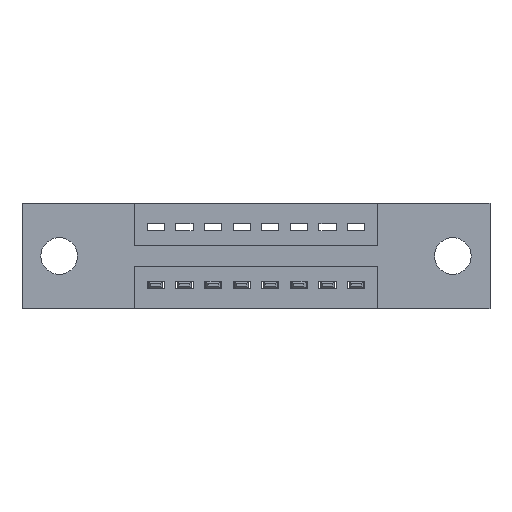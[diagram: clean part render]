
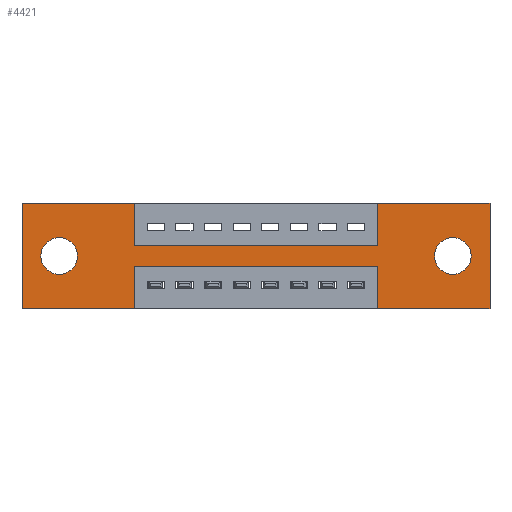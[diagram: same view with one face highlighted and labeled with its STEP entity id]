
A CAD part, front view. The second image highlights one B-rep face of the part: STEP entity #4421.
In plain terms, the highlighted planar face has unit normal (0, -1, 0).
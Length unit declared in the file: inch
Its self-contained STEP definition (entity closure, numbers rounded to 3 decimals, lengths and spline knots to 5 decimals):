
#73 = EDGE_CURVE ( 'NONE', #10025, #8509, #4733, .T. ) ;
#220 = LINE ( 'NONE', #9165, #4838 ) ;
#269 = VECTOR ( 'NONE', #8392, 39.37008 ) ;
#322 = VERTEX_POINT ( 'NONE', #3657 ) ;
#391 = CARTESIAN_POINT ( 'NONE',  ( 1.505, 0., -0.121 ) ) ;
#404 = DIRECTION ( 'NONE',  ( 0., 0., -1. ) ) ;
#452 = CARTESIAN_POINT ( 'NONE',  ( 0.3925, 0., -0.22 ) ) ;
#542 = CARTESIAN_POINT ( 'NONE',  ( 1.505, 0., -0.185 ) ) ;
#641 = DIRECTION ( 'NONE',  ( 0., 1., 0. ) ) ;
#740 = DIRECTION ( 'NONE',  ( 0., 1., 0. ) ) ;
#935 = CARTESIAN_POINT ( 'NONE',  ( 0.13, 0., -0.185 ) ) ;
#947 = EDGE_LOOP ( 'NONE', ( #5381, #6802 ) ) ;
#1046 = EDGE_CURVE ( 'NONE', #4358, #2756, #7135, .T. ) ;
#1125 = DIRECTION ( 'NONE',  ( 1., 0., 0. ) ) ;
#1167 = ORIENTED_EDGE ( 'NONE', *, *, #4762, .F. ) ;
#1325 = EDGE_LOOP ( 'NONE', ( #3595, #9137, #6911, #9579, #1167, #4138, #9545, #3908, #5271, #3804, #4996, #5662 ) ) ;
#1369 = LINE ( 'NONE', #5458, #9127 ) ;
#1416 = CARTESIAN_POINT ( 'NONE',  ( 1.635, 0., 0. ) ) ;
#1525 = CARTESIAN_POINT ( 'NONE',  ( 0.3925, 0., 0. ) ) ;
#1591 = VERTEX_POINT ( 'NONE', #1525 ) ;
#1653 = VERTEX_POINT ( 'NONE', #391 ) ;
#1808 = AXIS2_PLACEMENT_3D ( 'NONE', #6473, #740, #6333 ) ;
#1880 = VERTEX_POINT ( 'NONE', #6516 ) ;
#2045 = LINE ( 'NONE', #452, #269 ) ;
#2069 = FACE_BOUND ( 'NONE', #8489, .T. ) ;
#2163 = LINE ( 'NONE', #7488, #8297 ) ;
#2205 = VERTEX_POINT ( 'NONE', #9618 ) ;
#2238 = DIRECTION ( 'NONE',  ( 0., 0., -1. ) ) ;
#2328 = VECTOR ( 'NONE', #7051, 39.37008 ) ;
#2330 = VERTEX_POINT ( 'NONE', #2589 ) ;
#2357 = VERTEX_POINT ( 'NONE', #2485 ) ;
#2485 = CARTESIAN_POINT ( 'NONE',  ( 1.635, 0., 0. ) ) ;
#2589 = CARTESIAN_POINT ( 'NONE',  ( 1.2425, 0., -0.15 ) ) ;
#2756 = VERTEX_POINT ( 'NONE', #9376 ) ;
#2794 = DIRECTION ( 'NONE',  ( -1., 0., 0. ) ) ;
#2967 = CARTESIAN_POINT ( 'NONE',  ( 0.3925, 0., -0.22 ) ) ;
#3181 = VECTOR ( 'NONE', #4890, 39.37008 ) ;
#3317 = DIRECTION ( 'NONE',  ( 0., 0., -1. ) ) ;
#3364 = CARTESIAN_POINT ( 'NONE',  ( 0., 0., 0. ) ) ;
#3390 = VECTOR ( 'NONE', #5902, 39.37008 ) ;
#3561 = CARTESIAN_POINT ( 'NONE',  ( 1.2425, 0., 0. ) ) ;
#3593 = CARTESIAN_POINT ( 'NONE',  ( 0., 0., 0. ) ) ;
#3595 = ORIENTED_EDGE ( 'NONE', *, *, #5551, .F. ) ;
#3657 = CARTESIAN_POINT ( 'NONE',  ( 1.635, 0., -0.37 ) ) ;
#3683 = CIRCLE ( 'NONE', #6192, 0.064 ) ;
#3721 = EDGE_CURVE ( 'NONE', #8509, #10025, #3811, .T. ) ;
#3778 = DIRECTION ( 'NONE',  ( -1., 0., 0. ) ) ;
#3804 = ORIENTED_EDGE ( 'NONE', *, *, #5001, .F. ) ;
#3811 = CIRCLE ( 'NONE', #4106, 0.064 ) ;
#3908 = ORIENTED_EDGE ( 'NONE', *, *, #9086, .F. ) ;
#3918 = FACE_OUTER_BOUND ( 'NONE', #1325, .T. ) ;
#4019 = VERTEX_POINT ( 'NONE', #8410 ) ;
#4049 = CARTESIAN_POINT ( 'NONE',  ( 0.3925, 0., 0. ) ) ;
#4064 = EDGE_CURVE ( 'NONE', #1653, #2205, #3683, .T. ) ;
#4106 = AXIS2_PLACEMENT_3D ( 'NONE', #4189, #6502, #6469 ) ;
#4138 = ORIENTED_EDGE ( 'NONE', *, *, #4409, .F. ) ;
#4189 = CARTESIAN_POINT ( 'NONE',  ( 0.13, 0., -0.185 ) ) ;
#4358 = VERTEX_POINT ( 'NONE', #5880 ) ;
#4379 = PLANE ( 'NONE',  #8015 ) ;
#4399 = ORIENTED_EDGE ( 'NONE', *, *, #3721, .T. ) ;
#4409 = EDGE_CURVE ( 'NONE', #8389, #2357, #7200, .T. ) ;
#4418 = FACE_BOUND ( 'NONE', #947, .T. ) ;
#4421 = ADVANCED_FACE ( 'NONE', ( #4418, #2069, #3918 ), #4379, .T. ) ;
#4439 = CARTESIAN_POINT ( 'NONE',  ( 0., 0., -0.37 ) ) ;
#4633 = CARTESIAN_POINT ( 'NONE',  ( 0.13, 0., -0.121 ) ) ;
#4733 = CIRCLE ( 'NONE', #6994, 0.064 ) ;
#4762 = EDGE_CURVE ( 'NONE', #2357, #322, #7579, .T. ) ;
#4838 = VECTOR ( 'NONE', #2794, 39.37008 ) ;
#4857 = LINE ( 'NONE', #6743, #8770 ) ;
#4883 = VERTEX_POINT ( 'NONE', #5802 ) ;
#4890 = DIRECTION ( 'NONE',  ( 1., 0., 0. ) ) ;
#4996 = ORIENTED_EDGE ( 'NONE', *, *, #9316, .F. ) ;
#5001 = EDGE_CURVE ( 'NONE', #4019, #1591, #7060, .T. ) ;
#5130 = CARTESIAN_POINT ( 'NONE',  ( 0.13, 0., -0.249 ) ) ;
#5191 = DIRECTION ( 'NONE',  ( 0., -1., 0. ) ) ;
#5271 = ORIENTED_EDGE ( 'NONE', *, *, #6342, .F. ) ;
#5311 = LINE ( 'NONE', #7017, #2328 ) ;
#5313 = EDGE_CURVE ( 'NONE', #4883, #8506, #2045, .T. ) ;
#5381 = ORIENTED_EDGE ( 'NONE', *, *, #4064, .T. ) ;
#5427 = VECTOR ( 'NONE', #2238, 39.37008 ) ;
#5458 = CARTESIAN_POINT ( 'NONE',  ( 0., 0., 0. ) ) ;
#5465 = DIRECTION ( 'NONE',  ( 0., 0., -1. ) ) ;
#5551 = EDGE_CURVE ( 'NONE', #8506, #4358, #2163, .T. ) ;
#5662 = ORIENTED_EDGE ( 'NONE', *, *, #1046, .F. ) ;
#5802 = CARTESIAN_POINT ( 'NONE',  ( 1.2425, 0., -0.22 ) ) ;
#5839 = CIRCLE ( 'NONE', #1808, 0.064 ) ;
#5880 = CARTESIAN_POINT ( 'NONE',  ( 0.3925, 0., -0.37 ) ) ;
#5902 = DIRECTION ( 'NONE',  ( 0., 0., 1. ) ) ;
#6192 = AXIS2_PLACEMENT_3D ( 'NONE', #542, #641, #5465 ) ;
#6194 = VECTOR ( 'NONE', #3317, 39.37008 ) ;
#6196 = ORIENTED_EDGE ( 'NONE', *, *, #73, .T. ) ;
#6304 = EDGE_CURVE ( 'NONE', #1880, #4883, #5311, .T. ) ;
#6333 = DIRECTION ( 'NONE',  ( 0., 0., -1. ) ) ;
#6342 = EDGE_CURVE ( 'NONE', #1591, #8893, #9196, .T. ) ;
#6469 = DIRECTION ( 'NONE',  ( 0., 0., 1. ) ) ;
#6473 = CARTESIAN_POINT ( 'NONE',  ( 1.505, 0., -0.185 ) ) ;
#6502 = DIRECTION ( 'NONE',  ( 0., 1., 0. ) ) ;
#6516 = CARTESIAN_POINT ( 'NONE',  ( 1.2425, 0., -0.37 ) ) ;
#6611 = DIRECTION ( 'NONE',  ( 0., 1., 0. ) ) ;
#6743 = CARTESIAN_POINT ( 'NONE',  ( 0.3925, 0., -0.15 ) ) ;
#6802 = ORIENTED_EDGE ( 'NONE', *, *, #9712, .T. ) ;
#6911 = ORIENTED_EDGE ( 'NONE', *, *, #6304, .F. ) ;
#6994 = AXIS2_PLACEMENT_3D ( 'NONE', #935, #6611, #7424 ) ;
#7017 = CARTESIAN_POINT ( 'NONE',  ( 1.2425, 0., -0.37 ) ) ;
#7051 = DIRECTION ( 'NONE',  ( 0., 0., 1. ) ) ;
#7060 = LINE ( 'NONE', #3364, #3181 ) ;
#7135 = LINE ( 'NONE', #4439, #10030 ) ;
#7200 = LINE ( 'NONE', #3593, #10096 ) ;
#7424 = DIRECTION ( 'NONE',  ( 0., 0., 1. ) ) ;
#7488 = CARTESIAN_POINT ( 'NONE',  ( 0.3925, 0., -0.37 ) ) ;
#7579 = LINE ( 'NONE', #1416, #5427 ) ;
#8015 = AXIS2_PLACEMENT_3D ( 'NONE', #10017, #5191, #404 ) ;
#8297 = VECTOR ( 'NONE', #9150, 39.37008 ) ;
#8302 = EDGE_CURVE ( 'NONE', #2330, #8389, #8910, .T. ) ;
#8389 = VERTEX_POINT ( 'NONE', #3561 ) ;
#8392 = DIRECTION ( 'NONE',  ( -1., 0., 0. ) ) ;
#8410 = CARTESIAN_POINT ( 'NONE',  ( 0., 0., 0. ) ) ;
#8464 = CARTESIAN_POINT ( 'NONE',  ( 0.3925, 0., -0.15 ) ) ;
#8489 = EDGE_LOOP ( 'NONE', ( #4399, #6196 ) ) ;
#8506 = VERTEX_POINT ( 'NONE', #2967 ) ;
#8509 = VERTEX_POINT ( 'NONE', #4633 ) ;
#8540 = DIRECTION ( 'NONE',  ( 0., 0., 1. ) ) ;
#8770 = VECTOR ( 'NONE', #1125, 39.37008 ) ;
#8893 = VERTEX_POINT ( 'NONE', #8464 ) ;
#8910 = LINE ( 'NONE', #10005, #3390 ) ;
#9086 = EDGE_CURVE ( 'NONE', #8893, #2330, #4857, .T. ) ;
#9127 = VECTOR ( 'NONE', #8540, 39.37008 ) ;
#9137 = ORIENTED_EDGE ( 'NONE', *, *, #5313, .F. ) ;
#9150 = DIRECTION ( 'NONE',  ( 0., 0., -1. ) ) ;
#9165 = CARTESIAN_POINT ( 'NONE',  ( 0., 0., -0.37 ) ) ;
#9188 = DIRECTION ( 'NONE',  ( 1., 0., 0. ) ) ;
#9196 = LINE ( 'NONE', #4049, #6194 ) ;
#9316 = EDGE_CURVE ( 'NONE', #2756, #4019, #1369, .T. ) ;
#9376 = CARTESIAN_POINT ( 'NONE',  ( 0., 0., -0.37 ) ) ;
#9545 = ORIENTED_EDGE ( 'NONE', *, *, #8302, .F. ) ;
#9579 = ORIENTED_EDGE ( 'NONE', *, *, #9986, .F. ) ;
#9618 = CARTESIAN_POINT ( 'NONE',  ( 1.505, 0., -0.249 ) ) ;
#9712 = EDGE_CURVE ( 'NONE', #2205, #1653, #5839, .T. ) ;
#9986 = EDGE_CURVE ( 'NONE', #322, #1880, #220, .T. ) ;
#10005 = CARTESIAN_POINT ( 'NONE',  ( 1.2425, 0., 0. ) ) ;
#10017 = CARTESIAN_POINT ( 'NONE',  ( 0., 0., -0.37 ) ) ;
#10025 = VERTEX_POINT ( 'NONE', #5130 ) ;
#10030 = VECTOR ( 'NONE', #3778, 39.37008 ) ;
#10096 = VECTOR ( 'NONE', #9188, 39.37008 ) ;
